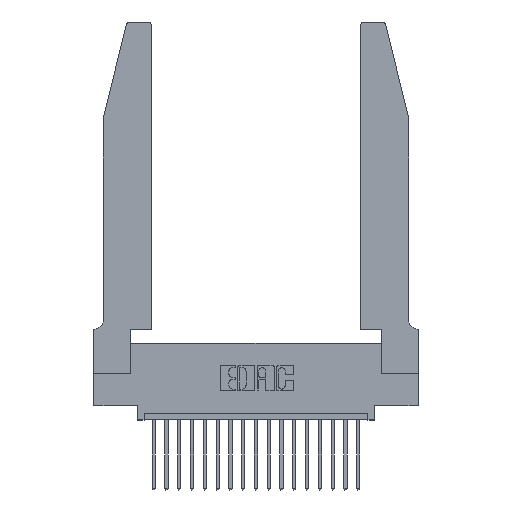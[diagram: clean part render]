
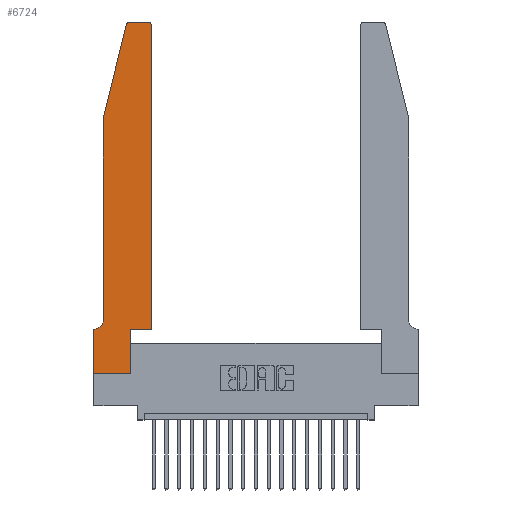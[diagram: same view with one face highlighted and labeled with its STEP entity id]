
A CAD part, top view. The second image highlights one B-rep face of the part: STEP entity #6724.
In plain terms, the highlighted planar face has unit normal (0, 0, 1).
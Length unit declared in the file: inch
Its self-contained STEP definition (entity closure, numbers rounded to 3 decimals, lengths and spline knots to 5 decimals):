
#279 = CARTESIAN_POINT ( 'NONE',  ( 0.2865, 0., 0.37 ) ) ;
#647 = CARTESIAN_POINT ( 'NONE',  ( 0.0755, 0.35, 0.37 ) ) ;
#768 = AXIS2_PLACEMENT_3D ( 'NONE', #13016, #3237, #17784 ) ;
#1225 = CARTESIAN_POINT ( 'NONE',  ( 0.0755, 2., 0.37 ) ) ;
#1443 = CARTESIAN_POINT ( 'NONE',  ( 0.4505, 0.35, 0.37 ) ) ;
#1610 = EDGE_CURVE ( 'NONE', #1820, #8118, #17816, .T. ) ;
#1820 = VERTEX_POINT ( 'NONE', #10477 ) ;
#1894 = VECTOR ( 'NONE', #8026, 39.37008 ) ;
#1900 = VERTEX_POINT ( 'NONE', #18563 ) ;
#2027 = EDGE_CURVE ( 'NONE', #12735, #12130, #17276, .T. ) ;
#2136 = DIRECTION ( 'NONE',  ( 0., 0., 1. ) ) ;
#2409 = LINE ( 'NONE', #14520, #1894 ) ;
#2626 = CARTESIAN_POINT ( 'NONE',  ( 0.4505, 0.35, 0.37 ) ) ;
#2632 = DIRECTION ( 'NONE',  ( 0., -1., 0. ) ) ;
#2790 = DIRECTION ( 'NONE',  ( 0., 1., 0. ) ) ;
#2892 = VECTOR ( 'NONE', #11828, 39.37008 ) ;
#2956 = VERTEX_POINT ( 'NONE', #15831 ) ;
#3237 = DIRECTION ( 'NONE',  ( 0., 0., 1. ) ) ;
#3461 = CARTESIAN_POINT ( 'NONE',  ( 0.284, 2.72, 0.37 ) ) ;
#3753 = VECTOR ( 'NONE', #2790, 39.37008 ) ;
#3996 = LINE ( 'NONE', #647, #14456 ) ;
#4078 = CARTESIAN_POINT ( 'NONE',  ( 0.0055, 0.42, 0.37 ) ) ;
#4208 = EDGE_CURVE ( 'NONE', #8118, #12305, #15150, .T. ) ;
#4476 = CARTESIAN_POINT ( 'NONE',  ( 0.284, 2.75, 0.37 ) ) ;
#4808 = EDGE_CURVE ( 'NONE', #12130, #16756, #19422, .T. ) ;
#5491 = CARTESIAN_POINT ( 'NONE',  ( 0.2605, 2.75, 0.37 ) ) ;
#5677 = CIRCLE ( 'NONE', #10466, 0.07 ) ;
#5748 = CARTESIAN_POINT ( 'NONE',  ( 0.4505, 2.72, 0.37 ) ) ;
#5847 = EDGE_CURVE ( 'NONE', #2956, #12735, #14814, .T. ) ;
#6309 = EDGE_CURVE ( 'NONE', #16917, #2956, #14127, .T. ) ;
#6331 = ORIENTED_EDGE ( 'NONE', *, *, #6309, .T. ) ;
#6487 = VECTOR ( 'NONE', #10988, 39.37008 ) ;
#6724 = ADVANCED_FACE ( 'NONE', ( #11545 ), #10118, .T. ) ;
#7293 = DIRECTION ( 'NONE',  ( -1., 0., 0. ) ) ;
#7608 = EDGE_CURVE ( 'NONE', #9539, #1900, #14809, .T. ) ;
#8026 = DIRECTION ( 'NONE',  ( 1., 0., 0. ) ) ;
#8104 = DIRECTION ( 'NONE',  ( -0.239, -0.971, 0. ) ) ;
#8118 = VERTEX_POINT ( 'NONE', #15594 ) ;
#8480 = ORIENTED_EDGE ( 'NONE', *, *, #14947, .T. ) ;
#8715 = VECTOR ( 'NONE', #2632, 39.37008 ) ;
#8844 = ORIENTED_EDGE ( 'NONE', *, *, #13675, .T. ) ;
#8947 = ORIENTED_EDGE ( 'NONE', *, *, #2027, .T. ) ;
#9348 = VERTEX_POINT ( 'NONE', #17580 ) ;
#9355 = ORIENTED_EDGE ( 'NONE', *, *, #5847, .T. ) ;
#9539 = VERTEX_POINT ( 'NONE', #16519 ) ;
#10118 = PLANE ( 'NONE',  #11914 ) ;
#10189 = ORIENTED_EDGE ( 'NONE', *, *, #4208, .T. ) ;
#10247 = ORIENTED_EDGE ( 'NONE', *, *, #19485, .T. ) ;
#10466 = AXIS2_PLACEMENT_3D ( 'NONE', #4078, #18538, #7293 ) ;
#10477 = CARTESIAN_POINT ( 'NONE',  ( 0.25487, 2.72718, 0.37 ) ) ;
#10614 = ORIENTED_EDGE ( 'NONE', *, *, #7608, .T. ) ;
#10857 = VERTEX_POINT ( 'NONE', #4476 ) ;
#10988 = DIRECTION ( 'NONE',  ( 0., -1., 0. ) ) ;
#11142 = CIRCLE ( 'NONE', #18441, 0.03 ) ;
#11545 = FACE_OUTER_BOUND ( 'NONE', #14678, .T. ) ;
#11602 = EDGE_CURVE ( 'NONE', #16756, #10857, #12906, .T. ) ;
#11604 = DIRECTION ( 'NONE',  ( 1., 0., 0. ) ) ;
#11702 = CARTESIAN_POINT ( 'NONE',  ( 0., 0.35, 0.37 ) ) ;
#11828 = DIRECTION ( 'NONE',  ( 0., 1., 0. ) ) ;
#11837 = DIRECTION ( 'NONE',  ( 1., 0., 0. ) ) ;
#11914 = AXIS2_PLACEMENT_3D ( 'NONE', #11702, #11915, #11837 ) ;
#11915 = DIRECTION ( 'NONE',  ( 0., 0., 1. ) ) ;
#12130 = VERTEX_POINT ( 'NONE', #5748 ) ;
#12248 = DIRECTION ( 'NONE',  ( -1., 0., 0. ) ) ;
#12305 = VERTEX_POINT ( 'NONE', #13442 ) ;
#12735 = VERTEX_POINT ( 'NONE', #13897 ) ;
#12906 = LINE ( 'NONE', #5491, #21009 ) ;
#13016 = CARTESIAN_POINT ( 'NONE',  ( 0.4205, 2.72, 0.37 ) ) ;
#13442 = CARTESIAN_POINT ( 'NONE',  ( 0.0755, 0.42, 0.37 ) ) ;
#13522 = EDGE_CURVE ( 'NONE', #10857, #1820, #11142, .T. ) ;
#13675 = EDGE_CURVE ( 'NONE', #9348, #9539, #3996, .T. ) ;
#13737 = VECTOR ( 'NONE', #8104, 39.37008 ) ;
#13897 = CARTESIAN_POINT ( 'NONE',  ( 0.4505, 0.35, 0.37 ) ) ;
#14029 = ORIENTED_EDGE ( 'NONE', *, *, #13522, .T. ) ;
#14127 = LINE ( 'NONE', #17812, #2892 ) ;
#14456 = VECTOR ( 'NONE', #12248, 39.37008 ) ;
#14520 = CARTESIAN_POINT ( 'NONE',  ( 0., 0., 0.37 ) ) ;
#14678 = EDGE_LOOP ( 'NONE', ( #19055, #14029, #17477, #10189, #10247, #8844, #10614, #8480, #6331, #9355, #8947, #15472 ) ) ;
#14809 = LINE ( 'NONE', #15609, #8715 ) ;
#14814 = LINE ( 'NONE', #2626, #16595 ) ;
#14947 = EDGE_CURVE ( 'NONE', #1900, #16917, #2409, .T. ) ;
#15150 = LINE ( 'NONE', #20706, #6487 ) ;
#15342 = DIRECTION ( 'NONE',  ( -1., 0., 0. ) ) ;
#15472 = ORIENTED_EDGE ( 'NONE', *, *, #4808, .T. ) ;
#15594 = CARTESIAN_POINT ( 'NONE',  ( 0.0755, 2., 0.37 ) ) ;
#15609 = CARTESIAN_POINT ( 'NONE',  ( 0., 0., 0.37 ) ) ;
#15831 = CARTESIAN_POINT ( 'NONE',  ( 0.2865, 0.35, 0.37 ) ) ;
#16173 = DIRECTION ( 'NONE',  ( 1., 0., 0. ) ) ;
#16386 = CARTESIAN_POINT ( 'NONE',  ( 0.4205, 2.75, 0.37 ) ) ;
#16519 = CARTESIAN_POINT ( 'NONE',  ( 0., 0.35, 0.37 ) ) ;
#16595 = VECTOR ( 'NONE', #16173, 39.37008 ) ;
#16756 = VERTEX_POINT ( 'NONE', #16386 ) ;
#16917 = VERTEX_POINT ( 'NONE', #279 ) ;
#17276 = LINE ( 'NONE', #1443, #3753 ) ;
#17477 = ORIENTED_EDGE ( 'NONE', *, *, #1610, .T. ) ;
#17580 = CARTESIAN_POINT ( 'NONE',  ( 0.0055, 0.35, 0.37 ) ) ;
#17784 = DIRECTION ( 'NONE',  ( 1., 0., 0. ) ) ;
#17812 = CARTESIAN_POINT ( 'NONE',  ( 0.2865, 0.35, 0.37 ) ) ;
#17816 = LINE ( 'NONE', #1225, #13737 ) ;
#18441 = AXIS2_PLACEMENT_3D ( 'NONE', #3461, #2136, #11604 ) ;
#18538 = DIRECTION ( 'NONE',  ( 0., 0., -1. ) ) ;
#18563 = CARTESIAN_POINT ( 'NONE',  ( 0., 0., 0.37 ) ) ;
#19055 = ORIENTED_EDGE ( 'NONE', *, *, #11602, .T. ) ;
#19422 = CIRCLE ( 'NONE', #768, 0.03 ) ;
#19485 = EDGE_CURVE ( 'NONE', #12305, #9348, #5677, .T. ) ;
#20706 = CARTESIAN_POINT ( 'NONE',  ( 0.0755, 2., 0.37 ) ) ;
#21009 = VECTOR ( 'NONE', #15342, 39.37008 ) ;
